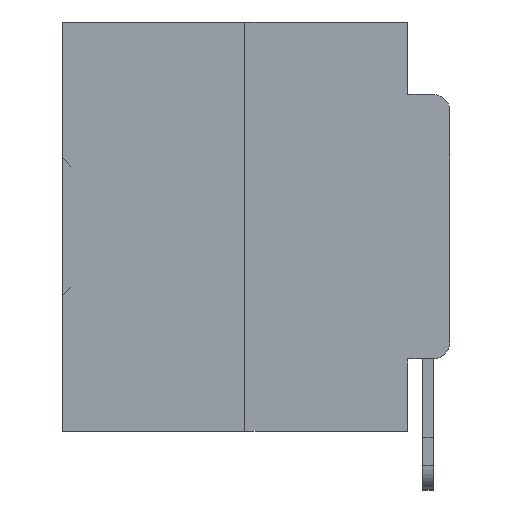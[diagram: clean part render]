
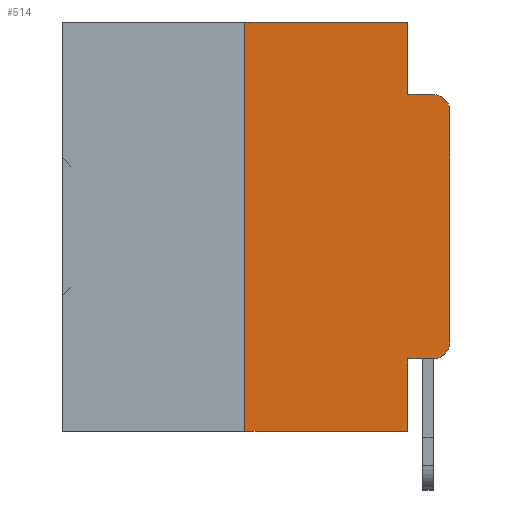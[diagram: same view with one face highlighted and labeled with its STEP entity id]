
A CAD part, left-side view. The second image highlights one B-rep face of the part: STEP entity #514.
In plain terms, the highlighted planar face has unit normal (-1, 0, 0).
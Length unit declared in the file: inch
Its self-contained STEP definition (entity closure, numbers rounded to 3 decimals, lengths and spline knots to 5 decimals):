
#52 = CARTESIAN_POINT ( 'NONE',  ( 0., 0.02, -0.0885 ) ) ;
#514 = ADVANCED_FACE ( 'NONE', ( #20660 ), #28575, .F. ) ;
#1130 = CARTESIAN_POINT ( 'NONE',  ( 0., 0.051, 0. ) ) ;
#1210 = CIRCLE ( 'NONE', #34881, 0.02 ) ;
#1571 = CARTESIAN_POINT ( 'NONE',  ( 0., 0.051, 0. ) ) ;
#1712 = DIRECTION ( 'NONE',  ( 0., 0., -1. ) ) ;
#2001 = CARTESIAN_POINT ( 'NONE',  ( 0., 0.25, 0. ) ) ;
#2342 = DIRECTION ( 'NONE',  ( 0., 0., 1. ) ) ;
#2638 = ORIENTED_EDGE ( 'NONE', *, *, #20439, .T. ) ;
#2842 = AXIS2_PLACEMENT_3D ( 'NONE', #13813, #31455, #13941 ) ;
#3125 = ORIENTED_EDGE ( 'NONE', *, *, #3409, .F. ) ;
#3409 = EDGE_CURVE ( 'NONE', #30330, #18364, #19564, .T. ) ;
#3638 = VERTEX_POINT ( 'NONE', #4100 ) ;
#4100 = CARTESIAN_POINT ( 'NONE',  ( 0., 0.051, -0.4115 ) ) ;
#4671 = EDGE_CURVE ( 'NONE', #18993, #18364, #5630, .T. ) ;
#5095 = CARTESIAN_POINT ( 'NONE',  ( 0., 0., -0.3915 ) ) ;
#5369 = LINE ( 'NONE', #33910, #36858 ) ;
#5447 = VERTEX_POINT ( 'NONE', #5095 ) ;
#5630 = CIRCLE ( 'NONE', #17037, 0.02 ) ;
#5661 = CARTESIAN_POINT ( 'NONE',  ( 0., 0.051, -0.4115 ) ) ;
#5796 = DIRECTION ( 'NONE',  ( 0., -1., 0. ) ) ;
#7999 = EDGE_CURVE ( 'NONE', #16121, #5447, #1210, .T. ) ;
#8208 = VECTOR ( 'NONE', #29591, 39.37008 ) ;
#8837 = CARTESIAN_POINT ( 'NONE',  ( 0., 0.02, -0.1085 ) ) ;
#9319 = LINE ( 'NONE', #14382, #31942 ) ;
#9475 = EDGE_CURVE ( 'NONE', #25740, #25568, #9319, .T. ) ;
#10722 = EDGE_CURVE ( 'NONE', #15895, #25740, #22488, .T. ) ;
#11334 = DIRECTION ( 'NONE',  ( -1., 0., 0. ) ) ;
#11658 = VECTOR ( 'NONE', #5796, 39.37008 ) ;
#11990 = DIRECTION ( 'NONE',  ( 0., 0., -1. ) ) ;
#12224 = EDGE_CURVE ( 'NONE', #15895, #38580, #5369, .T. ) ;
#13211 = VECTOR ( 'NONE', #21248, 39.37008 ) ;
#13746 = EDGE_CURVE ( 'NONE', #3638, #38580, #18542, .T. ) ;
#13813 = CARTESIAN_POINT ( 'NONE',  ( 0., 0.473, 0. ) ) ;
#13941 = DIRECTION ( 'NONE',  ( 0., 0., -1. ) ) ;
#14382 = CARTESIAN_POINT ( 'NONE',  ( 0., 0.473, 0. ) ) ;
#15895 = VERTEX_POINT ( 'NONE', #24334 ) ;
#16072 = CARTESIAN_POINT ( 'NONE',  ( 0., 0.051, -0.0885 ) ) ;
#16121 = VERTEX_POINT ( 'NONE', #16512 ) ;
#16280 = DIRECTION ( 'NONE',  ( 0., -1., 0. ) ) ;
#16364 = LINE ( 'NONE', #5661, #8208 ) ;
#16512 = CARTESIAN_POINT ( 'NONE',  ( 0., 0.02, -0.4115 ) ) ;
#16692 = ORIENTED_EDGE ( 'NONE', *, *, #21173, .T. ) ;
#17037 = AXIS2_PLACEMENT_3D ( 'NONE', #8837, #29594, #11990 ) ;
#17642 = VECTOR ( 'NONE', #1712, 39.37008 ) ;
#18236 = CARTESIAN_POINT ( 'NONE',  ( 0., 0., 0. ) ) ;
#18364 = VERTEX_POINT ( 'NONE', #52 ) ;
#18542 = LINE ( 'NONE', #37190, #17642 ) ;
#18993 = VERTEX_POINT ( 'NONE', #35378 ) ;
#19442 = ORIENTED_EDGE ( 'NONE', *, *, #37727, .F. ) ;
#19564 = LINE ( 'NONE', #29719, #11658 ) ;
#20343 = DIRECTION ( 'NONE',  ( 0., -1., 0. ) ) ;
#20439 = EDGE_CURVE ( 'NONE', #3638, #16121, #16364, .T. ) ;
#20660 = FACE_OUTER_BOUND ( 'NONE', #28301, .T. ) ;
#20706 = CARTESIAN_POINT ( 'NONE',  ( 0., 0.25, 0. ) ) ;
#21083 = LINE ( 'NONE', #18236, #13211 ) ;
#21173 = EDGE_CURVE ( 'NONE', #5447, #18993, #21083, .T. ) ;
#21248 = DIRECTION ( 'NONE',  ( 0., 0., 1. ) ) ;
#22488 = LINE ( 'NONE', #20706, #38687 ) ;
#23109 = ORIENTED_EDGE ( 'NONE', *, *, #12224, .T. ) ;
#24334 = CARTESIAN_POINT ( 'NONE',  ( 0., 0.25, -0.5 ) ) ;
#25568 = VERTEX_POINT ( 'NONE', #1130 ) ;
#25740 = VERTEX_POINT ( 'NONE', #2001 ) ;
#26308 = ORIENTED_EDGE ( 'NONE', *, *, #4671, .T. ) ;
#26759 = CARTESIAN_POINT ( 'NONE',  ( 0., 0.051, -0.5 ) ) ;
#27402 = VECTOR ( 'NONE', #31712, 39.37008 ) ;
#28106 = ORIENTED_EDGE ( 'NONE', *, *, #9475, .F. ) ;
#28301 = EDGE_LOOP ( 'NONE', ( #16692, #26308, #3125, #19442, #28106, #35755, #23109, #38398, #2638, #35331 ) ) ;
#28322 = LINE ( 'NONE', #1571, #27402 ) ;
#28575 = PLANE ( 'NONE',  #2842 ) ;
#28972 = CARTESIAN_POINT ( 'NONE',  ( 0., 0.02, -0.3915 ) ) ;
#29591 = DIRECTION ( 'NONE',  ( 0., -1., 0. ) ) ;
#29594 = DIRECTION ( 'NONE',  ( -1., 0., 0. ) ) ;
#29719 = CARTESIAN_POINT ( 'NONE',  ( 0., 0.051, -0.0885 ) ) ;
#30330 = VERTEX_POINT ( 'NONE', #16072 ) ;
#31455 = DIRECTION ( 'NONE',  ( 1., 0., 0. ) ) ;
#31712 = DIRECTION ( 'NONE',  ( 0., 0., -1. ) ) ;
#31849 = DIRECTION ( 'NONE',  ( 0., 0., -1. ) ) ;
#31942 = VECTOR ( 'NONE', #20343, 39.37008 ) ;
#33910 = CARTESIAN_POINT ( 'NONE',  ( 0., 0.473, -0.5 ) ) ;
#34881 = AXIS2_PLACEMENT_3D ( 'NONE', #28972, #11334, #31849 ) ;
#35331 = ORIENTED_EDGE ( 'NONE', *, *, #7999, .T. ) ;
#35378 = CARTESIAN_POINT ( 'NONE',  ( 0., 0., -0.1085 ) ) ;
#35755 = ORIENTED_EDGE ( 'NONE', *, *, #10722, .F. ) ;
#36858 = VECTOR ( 'NONE', #16280, 39.37008 ) ;
#37190 = CARTESIAN_POINT ( 'NONE',  ( 0., 0.051, 0. ) ) ;
#37727 = EDGE_CURVE ( 'NONE', #25568, #30330, #28322, .T. ) ;
#38398 = ORIENTED_EDGE ( 'NONE', *, *, #13746, .F. ) ;
#38580 = VERTEX_POINT ( 'NONE', #26759 ) ;
#38687 = VECTOR ( 'NONE', #2342, 39.37008 ) ;
